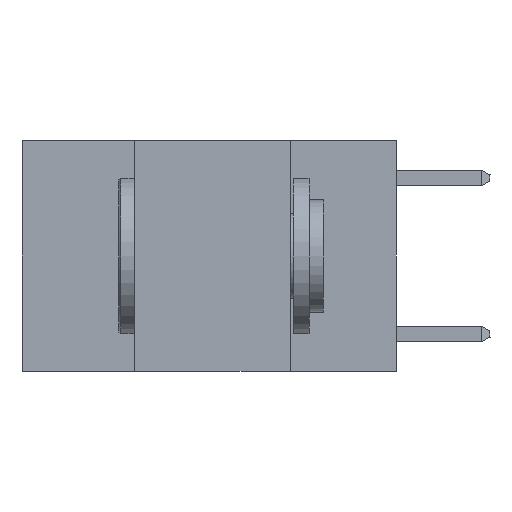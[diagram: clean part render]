
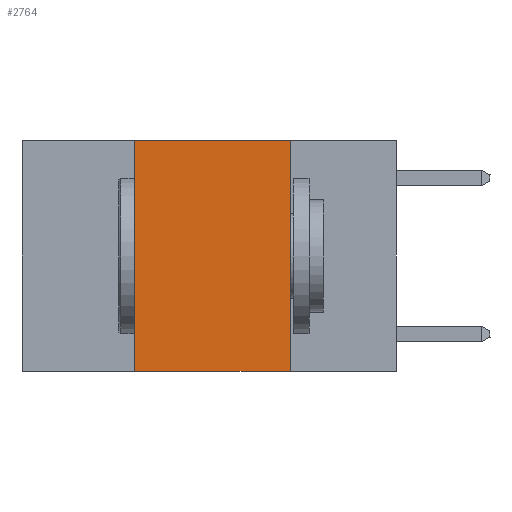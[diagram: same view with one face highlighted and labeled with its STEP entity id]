
A CAD part, left-side view. The second image highlights one B-rep face of the part: STEP entity #2764.
In plain terms, the highlighted planar face has unit normal (-1, 0, 0).
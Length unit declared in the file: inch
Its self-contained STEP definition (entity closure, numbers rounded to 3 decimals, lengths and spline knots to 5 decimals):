
#301 = LINE ( 'NONE', #10970, #854 ) ;
#753 = DIRECTION ( 'NONE',  ( 0., 0., -1. ) ) ;
#854 = VECTOR ( 'NONE', #24962, 39.37008 ) ;
#2322 = VERTEX_POINT ( 'NONE', #6996 ) ;
#2764 = ADVANCED_FACE ( 'NONE', ( #9006 ), #13053, .F. ) ;
#2781 = DIRECTION ( 'NONE',  ( 1., 0., 0. ) ) ;
#3140 = ORIENTED_EDGE ( 'NONE', *, *, #26051, .F. ) ;
#3221 = VECTOR ( 'NONE', #5606, 39.37008 ) ;
#3326 = CARTESIAN_POINT ( 'NONE',  ( 0., 0.6, 0. ) ) ;
#4375 = VERTEX_POINT ( 'NONE', #19376 ) ;
#5606 = DIRECTION ( 'NONE',  ( 0., -1., 0. ) ) ;
#6642 = EDGE_CURVE ( 'NONE', #17144, #4375, #301, .T. ) ;
#6786 = CARTESIAN_POINT ( 'NONE',  ( 0., 0.42, -0.37 ) ) ;
#6996 = CARTESIAN_POINT ( 'NONE',  ( 0., 0.17, -0.37 ) ) ;
#8332 = VECTOR ( 'NONE', #16292, 39.37008 ) ;
#9006 = FACE_OUTER_BOUND ( 'NONE', #26483, .T. ) ;
#9969 = LINE ( 'NONE', #14126, #8332 ) ;
#10256 = ORIENTED_EDGE ( 'NONE', *, *, #6642, .F. ) ;
#10970 = CARTESIAN_POINT ( 'NONE',  ( 0., 0.42, 0. ) ) ;
#13053 = PLANE ( 'NONE',  #18454 ) ;
#14126 = CARTESIAN_POINT ( 'NONE',  ( 0., 0.17, 0. ) ) ;
#15225 = CARTESIAN_POINT ( 'NONE',  ( 0., 0.17, 0. ) ) ;
#16292 = DIRECTION ( 'NONE',  ( 0., 0., -1. ) ) ;
#17144 = VERTEX_POINT ( 'NONE', #6786 ) ;
#17189 = EDGE_CURVE ( 'NONE', #17144, #2322, #24440, .T. ) ;
#18147 = CARTESIAN_POINT ( 'NONE',  ( 0., 0.6, -0.37 ) ) ;
#18454 = AXIS2_PLACEMENT_3D ( 'NONE', #21249, #2781, #753 ) ;
#18533 = VECTOR ( 'NONE', #26180, 39.37008 ) ;
#19376 = CARTESIAN_POINT ( 'NONE',  ( 0., 0.42, 0. ) ) ;
#21249 = CARTESIAN_POINT ( 'NONE',  ( 0., 0.6, 0. ) ) ;
#21345 = EDGE_CURVE ( 'NONE', #25523, #2322, #9969, .T. ) ;
#22662 = ORIENTED_EDGE ( 'NONE', *, *, #21345, .F. ) ;
#23846 = ORIENTED_EDGE ( 'NONE', *, *, #17189, .T. ) ;
#24440 = LINE ( 'NONE', #18147, #18533 ) ;
#24962 = DIRECTION ( 'NONE',  ( 0., 0., 1. ) ) ;
#25523 = VERTEX_POINT ( 'NONE', #15225 ) ;
#25555 = LINE ( 'NONE', #3326, #3221 ) ;
#26051 = EDGE_CURVE ( 'NONE', #4375, #25523, #25555, .T. ) ;
#26180 = DIRECTION ( 'NONE',  ( 0., -1., 0. ) ) ;
#26483 = EDGE_LOOP ( 'NONE', ( #22662, #3140, #10256, #23846 ) ) ;
